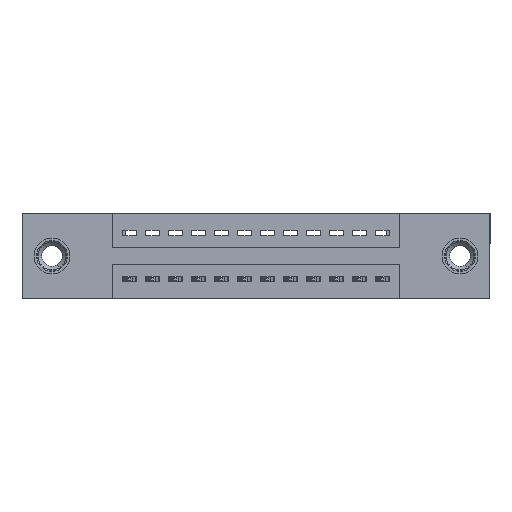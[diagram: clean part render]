
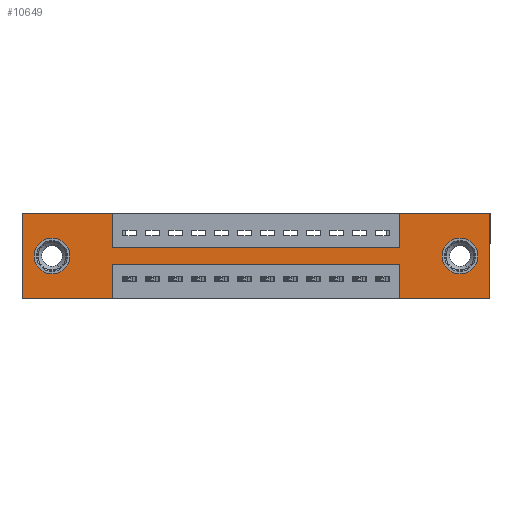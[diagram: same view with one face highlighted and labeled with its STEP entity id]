
A CAD part, front view. The second image highlights one B-rep face of the part: STEP entity #10649.
In plain terms, the highlighted planar face has unit normal (0, -1, 0).
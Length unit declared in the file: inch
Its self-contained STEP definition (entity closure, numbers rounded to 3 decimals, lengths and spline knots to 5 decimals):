
#8 = EDGE_CURVE ( 'NONE', #1671, #5551, #8645, .T. ) ;
#72 = VERTEX_POINT ( 'NONE', #15788 ) ;
#236 = EDGE_CURVE ( 'NONE', #10115, #753, #7368, .T. ) ;
#463 = CARTESIAN_POINT ( 'NONE',  ( 1.6425, 0., -0.15 ) ) ;
#576 = VECTOR ( 'NONE', #10908, 39.37008 ) ;
#753 = VERTEX_POINT ( 'NONE', #5898 ) ;
#847 = DIRECTION ( 'NONE',  ( 0., 0., -1. ) ) ;
#851 = AXIS2_PLACEMENT_3D ( 'NONE', #15909, #10396, #4878 ) ;
#895 = CARTESIAN_POINT ( 'NONE',  ( 0., 0., -0.37 ) ) ;
#972 = EDGE_CURVE ( 'NONE', #5551, #5021, #1602, .T. ) ;
#994 = VECTOR ( 'NONE', #10281, 39.37008 ) ;
#1027 = DIRECTION ( 'NONE',  ( 0., 0., 1. ) ) ;
#1050 = CARTESIAN_POINT ( 'NONE',  ( 0., 0., 0. ) ) ;
#1127 = DIRECTION ( 'NONE',  ( 1., 0., 0. ) ) ;
#1193 = EDGE_LOOP ( 'NONE', ( #7251, #10543 ) ) ;
#1219 = CARTESIAN_POINT ( 'NONE',  ( 1.6425, 0., -0.37 ) ) ;
#1265 = CARTESIAN_POINT ( 'NONE',  ( 2.035, 0., 0. ) ) ;
#1431 = EDGE_CURVE ( 'NONE', #10255, #7302, #11962, .T. ) ;
#1513 = CIRCLE ( 'NONE', #8365, 0.078 ) ;
#1602 = LINE ( 'NONE', #13289, #9368 ) ;
#1607 = CARTESIAN_POINT ( 'NONE',  ( 0.3925, 0., -0.22 ) ) ;
#1629 = DIRECTION ( 'NONE',  ( 0., 0., -1. ) ) ;
#1671 = VERTEX_POINT ( 'NONE', #1607 ) ;
#1857 = CARTESIAN_POINT ( 'NONE',  ( 0.3925, 0., -0.15 ) ) ;
#2157 = DIRECTION ( 'NONE',  ( -1., 0., 0. ) ) ;
#2162 = CARTESIAN_POINT ( 'NONE',  ( 2.035, 0., -0.37 ) ) ;
#2375 = CARTESIAN_POINT ( 'NONE',  ( 0.3925, 0., 0. ) ) ;
#2471 = CARTESIAN_POINT ( 'NONE',  ( 0.3925, 0., 0. ) ) ;
#2520 = VERTEX_POINT ( 'NONE', #12891 ) ;
#2825 = EDGE_CURVE ( 'NONE', #72, #7455, #12342, .T. ) ;
#3620 = LINE ( 'NONE', #6132, #994 ) ;
#3684 = VERTEX_POINT ( 'NONE', #17664 ) ;
#3915 = CARTESIAN_POINT ( 'NONE',  ( 2.035, 0., 0. ) ) ;
#4039 = ORIENTED_EDGE ( 'NONE', *, *, #7783, .F. ) ;
#4108 = AXIS2_PLACEMENT_3D ( 'NONE', #16179, #7982, #17430 ) ;
#4160 = CARTESIAN_POINT ( 'NONE',  ( 0., 0., -0.37 ) ) ;
#4203 = ORIENTED_EDGE ( 'NONE', *, *, #5584, .F. ) ;
#4338 = CARTESIAN_POINT ( 'NONE',  ( 0.3925, 0., -0.37 ) ) ;
#4361 = VECTOR ( 'NONE', #10594, 39.37008 ) ;
#4567 = ORIENTED_EDGE ( 'NONE', *, *, #8359, .T. ) ;
#4582 = DIRECTION ( 'NONE',  ( 0., -1., 0. ) ) ;
#4834 = VECTOR ( 'NONE', #16529, 39.37008 ) ;
#4850 = ORIENTED_EDGE ( 'NONE', *, *, #2825, .F. ) ;
#4878 = DIRECTION ( 'NONE',  ( 0., 0., -1. ) ) ;
#4934 = DIRECTION ( 'NONE',  ( 0., 0., 1. ) ) ;
#5021 = VERTEX_POINT ( 'NONE', #895 ) ;
#5147 = VERTEX_POINT ( 'NONE', #1857 ) ;
#5203 = AXIS2_PLACEMENT_3D ( 'NONE', #17365, #9276, #1027 ) ;
#5546 = FACE_OUTER_BOUND ( 'NONE', #12308, .T. ) ;
#5551 = VERTEX_POINT ( 'NONE', #4338 ) ;
#5584 = EDGE_CURVE ( 'NONE', #7455, #1671, #16114, .T. ) ;
#5898 = CARTESIAN_POINT ( 'NONE',  ( 0.13, 0., -0.263 ) ) ;
#5947 = CARTESIAN_POINT ( 'NONE',  ( 0., 0., -0.37 ) ) ;
#6132 = CARTESIAN_POINT ( 'NONE',  ( 0.3925, 0., -0.15 ) ) ;
#6177 = CARTESIAN_POINT ( 'NONE',  ( 1.6425, 0., 0. ) ) ;
#6272 = VERTEX_POINT ( 'NONE', #9712 ) ;
#6296 = ORIENTED_EDGE ( 'NONE', *, *, #8118, .F. ) ;
#6592 = CARTESIAN_POINT ( 'NONE',  ( 0., 0., 0. ) ) ;
#6910 = DIRECTION ( 'NONE',  ( -1., 0., 0. ) ) ;
#6914 = EDGE_CURVE ( 'NONE', #7302, #5147, #13492, .T. ) ;
#7055 = LINE ( 'NONE', #6592, #576 ) ;
#7251 = ORIENTED_EDGE ( 'NONE', *, *, #14676, .T. ) ;
#7302 = VERTEX_POINT ( 'NONE', #2471 ) ;
#7368 = CIRCLE ( 'NONE', #5203, 0.078 ) ;
#7408 = ORIENTED_EDGE ( 'NONE', *, *, #9609, .F. ) ;
#7455 = VERTEX_POINT ( 'NONE', #7748 ) ;
#7592 = ORIENTED_EDGE ( 'NONE', *, *, #8, .F. ) ;
#7748 = CARTESIAN_POINT ( 'NONE',  ( 1.6425, 0., -0.22 ) ) ;
#7783 = EDGE_CURVE ( 'NONE', #10593, #72, #16792, .T. ) ;
#7982 = DIRECTION ( 'NONE',  ( 0., 1., 0. ) ) ;
#8098 = ORIENTED_EDGE ( 'NONE', *, *, #6914, .F. ) ;
#8118 = EDGE_CURVE ( 'NONE', #2520, #16385, #15955, .T. ) ;
#8359 = EDGE_CURVE ( 'NONE', #753, #10115, #8602, .T. ) ;
#8365 = AXIS2_PLACEMENT_3D ( 'NONE', #13607, #13725, #14979 ) ;
#8551 = VECTOR ( 'NONE', #847, 39.37008 ) ;
#8602 = CIRCLE ( 'NONE', #4108, 0.078 ) ;
#8645 = LINE ( 'NONE', #14071, #11669 ) ;
#8988 = VECTOR ( 'NONE', #4934, 39.37008 ) ;
#9030 = VECTOR ( 'NONE', #6910, 39.37008 ) ;
#9054 = VECTOR ( 'NONE', #1127, 39.37008 ) ;
#9262 = EDGE_CURVE ( 'NONE', #5021, #10255, #7055, .T. ) ;
#9276 = DIRECTION ( 'NONE',  ( 0., 1., 0. ) ) ;
#9330 = CIRCLE ( 'NONE', #851, 0.078 ) ;
#9368 = VECTOR ( 'NONE', #2157, 39.37008 ) ;
#9609 = EDGE_CURVE ( 'NONE', #15631, #2520, #12428, .T. ) ;
#9712 = CARTESIAN_POINT ( 'NONE',  ( 1.905, 0., -0.263 ) ) ;
#9918 = LINE ( 'NONE', #3915, #4361 ) ;
#10115 = VERTEX_POINT ( 'NONE', #15740 ) ;
#10255 = VERTEX_POINT ( 'NONE', #14264 ) ;
#10281 = DIRECTION ( 'NONE',  ( 1., 0., 0. ) ) ;
#10335 = EDGE_CURVE ( 'NONE', #5147, #15631, #3620, .T. ) ;
#10396 = DIRECTION ( 'NONE',  ( 0., 1., 0. ) ) ;
#10473 = DIRECTION ( 'NONE',  ( -1., 0., 0. ) ) ;
#10543 = ORIENTED_EDGE ( 'NONE', *, *, #13345, .T. ) ;
#10593 = VERTEX_POINT ( 'NONE', #2162 ) ;
#10594 = DIRECTION ( 'NONE',  ( 0., 0., -1. ) ) ;
#10648 = AXIS2_PLACEMENT_3D ( 'NONE', #5947, #4582, #1629 ) ;
#10649 = ADVANCED_FACE ( 'NONE', ( #14307, #15841, #5546 ), #13898, .T. ) ;
#10908 = DIRECTION ( 'NONE',  ( 0., 0., 1. ) ) ;
#11278 = ORIENTED_EDGE ( 'NONE', *, *, #236, .T. ) ;
#11399 = DIRECTION ( 'NONE',  ( 0., 0., -1. ) ) ;
#11669 = VECTOR ( 'NONE', #11399, 39.37008 ) ;
#11962 = LINE ( 'NONE', #14971, #12174 ) ;
#12174 = VECTOR ( 'NONE', #17648, 39.37008 ) ;
#12308 = EDGE_LOOP ( 'NONE', ( #7592, #4203, #4850, #4039, #12776, #6296, #7408, #16748, #8098, #16656, #14981, #12522 ) ) ;
#12342 = LINE ( 'NONE', #1219, #4834 ) ;
#12428 = LINE ( 'NONE', #6177, #8988 ) ;
#12522 = ORIENTED_EDGE ( 'NONE', *, *, #972, .F. ) ;
#12776 = ORIENTED_EDGE ( 'NONE', *, *, #16975, .F. ) ;
#12891 = CARTESIAN_POINT ( 'NONE',  ( 1.6425, 0., 0. ) ) ;
#12971 = EDGE_LOOP ( 'NONE', ( #11278, #4567 ) ) ;
#13289 = CARTESIAN_POINT ( 'NONE',  ( 0., 0., -0.37 ) ) ;
#13345 = EDGE_CURVE ( 'NONE', #6272, #3684, #1513, .T. ) ;
#13492 = LINE ( 'NONE', #2375, #8551 ) ;
#13607 = CARTESIAN_POINT ( 'NONE',  ( 1.905, 0., -0.185 ) ) ;
#13725 = DIRECTION ( 'NONE',  ( 0., 1., 0. ) ) ;
#13898 = PLANE ( 'NONE',  #10648 ) ;
#13905 = VECTOR ( 'NONE', #10473, 39.37008 ) ;
#14071 = CARTESIAN_POINT ( 'NONE',  ( 0.3925, 0., -0.37 ) ) ;
#14264 = CARTESIAN_POINT ( 'NONE',  ( 0., 0., 0. ) ) ;
#14307 = FACE_BOUND ( 'NONE', #1193, .T. ) ;
#14676 = EDGE_CURVE ( 'NONE', #3684, #6272, #9330, .T. ) ;
#14971 = CARTESIAN_POINT ( 'NONE',  ( 0., 0., 0. ) ) ;
#14979 = DIRECTION ( 'NONE',  ( 0., 0., -1. ) ) ;
#14981 = ORIENTED_EDGE ( 'NONE', *, *, #9262, .F. ) ;
#15631 = VERTEX_POINT ( 'NONE', #463 ) ;
#15740 = CARTESIAN_POINT ( 'NONE',  ( 0.13, 0., -0.107 ) ) ;
#15788 = CARTESIAN_POINT ( 'NONE',  ( 1.6425, 0., -0.37 ) ) ;
#15841 = FACE_BOUND ( 'NONE', #12971, .T. ) ;
#15909 = CARTESIAN_POINT ( 'NONE',  ( 1.905, 0., -0.185 ) ) ;
#15955 = LINE ( 'NONE', #1050, #9054 ) ;
#16114 = LINE ( 'NONE', #17258, #13905 ) ;
#16179 = CARTESIAN_POINT ( 'NONE',  ( 0.13, 0., -0.185 ) ) ;
#16385 = VERTEX_POINT ( 'NONE', #1265 ) ;
#16529 = DIRECTION ( 'NONE',  ( 0., 0., 1. ) ) ;
#16656 = ORIENTED_EDGE ( 'NONE', *, *, #1431, .F. ) ;
#16748 = ORIENTED_EDGE ( 'NONE', *, *, #10335, .F. ) ;
#16792 = LINE ( 'NONE', #4160, #9030 ) ;
#16975 = EDGE_CURVE ( 'NONE', #16385, #10593, #9918, .T. ) ;
#17258 = CARTESIAN_POINT ( 'NONE',  ( 0.3925, 0., -0.22 ) ) ;
#17365 = CARTESIAN_POINT ( 'NONE',  ( 0.13, 0., -0.185 ) ) ;
#17430 = DIRECTION ( 'NONE',  ( 0., 0., 1. ) ) ;
#17648 = DIRECTION ( 'NONE',  ( 1., 0., 0. ) ) ;
#17664 = CARTESIAN_POINT ( 'NONE',  ( 1.905, 0., -0.107 ) ) ;
